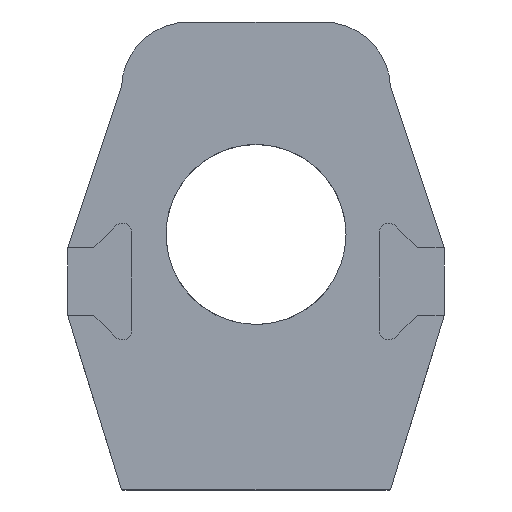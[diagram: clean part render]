
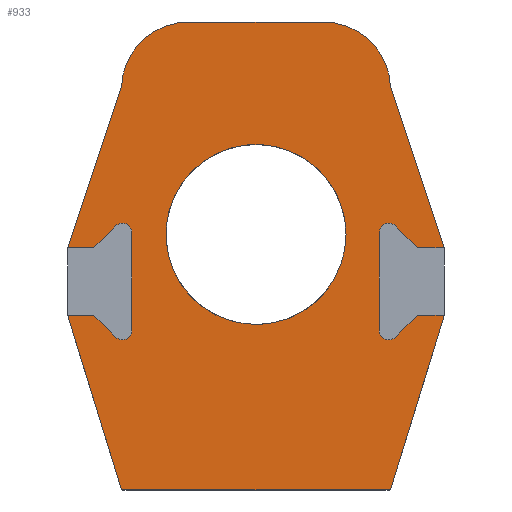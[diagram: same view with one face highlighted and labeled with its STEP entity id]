
A CAD part, front view. The second image highlights one B-rep face of the part: STEP entity #933.
In plain terms, the highlighted planar face has unit normal (0, -1, 0).
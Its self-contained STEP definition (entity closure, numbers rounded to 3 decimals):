
#19=ELLIPSE('',#1005,3.676,2.54);
#20=ELLIPSE('',#1012,3.676,2.54);
#58=FACE_BOUND('',#143,.T.);
#62=PLANE('',#1004);
#91=FACE_OUTER_BOUND('',#142,.T.);
#142=EDGE_LOOP('',(#667,#668,#669,#670,#671,#672,#673,#674,#675,#676,#677,
#678,#679,#680,#681,#682,#683,#684,#685,#686,#687,#688,#689,#690));
#143=EDGE_LOOP('',(#691,#692));
#202=LINE('',#1413,#299);
#203=LINE('',#1415,#300);
#204=LINE('',#1417,#301);
#205=LINE('',#1421,#302);
#206=LINE('',#1425,#303);
#207=LINE('',#1427,#304);
#208=LINE('',#1429,#305);
#209=LINE('',#1433,#306);
#210=LINE('',#1437,#307);
#211=LINE('',#1439,#308);
#212=LINE('',#1441,#309);
#213=LINE('',#1445,#310);
#214=LINE('',#1449,#311);
#215=LINE('',#1451,#312);
#216=LINE('',#1453,#313);
#217=LINE('',#1456,#314);
#299=VECTOR('',#1123,10.);
#300=VECTOR('',#1124,10.);
#301=VECTOR('',#1125,10.);
#302=VECTOR('',#1128,10.);
#303=VECTOR('',#1131,10.);
#304=VECTOR('',#1132,10.);
#305=VECTOR('',#1133,10.);
#306=VECTOR('',#1136,10.);
#307=VECTOR('',#1139,10.);
#308=VECTOR('',#1140,10.);
#309=VECTOR('',#1141,10.);
#310=VECTOR('',#1144,10.);
#311=VECTOR('',#1147,10.);
#312=VECTOR('',#1148,10.);
#313=VECTOR('',#1149,10.);
#314=VECTOR('',#1152,10.);
#393=CIRCLE('',#1006,0.889);
#394=CIRCLE('',#1007,0.889);
#395=CIRCLE('',#1008,6.35);
#396=CIRCLE('',#1009,6.35);
#397=CIRCLE('',#1010,0.889);
#398=CIRCLE('',#1011,0.889);
#399=CIRCLE('',#1013,8.5);
#400=CIRCLE('',#1014,8.5);
#426=VERTEX_POINT('',#1409);
#427=VERTEX_POINT('',#1410);
#428=VERTEX_POINT('',#1412);
#429=VERTEX_POINT('',#1414);
#430=VERTEX_POINT('',#1416);
#431=VERTEX_POINT('',#1418);
#432=VERTEX_POINT('',#1420);
#433=VERTEX_POINT('',#1422);
#434=VERTEX_POINT('',#1424);
#435=VERTEX_POINT('',#1426);
#436=VERTEX_POINT('',#1428);
#437=VERTEX_POINT('',#1430);
#438=VERTEX_POINT('',#1432);
#439=VERTEX_POINT('',#1434);
#440=VERTEX_POINT('',#1436);
#441=VERTEX_POINT('',#1438);
#442=VERTEX_POINT('',#1440);
#443=VERTEX_POINT('',#1442);
#444=VERTEX_POINT('',#1444);
#445=VERTEX_POINT('',#1446);
#446=VERTEX_POINT('',#1448);
#447=VERTEX_POINT('',#1450);
#448=VERTEX_POINT('',#1452);
#449=VERTEX_POINT('',#1454);
#450=VERTEX_POINT('',#1457);
#451=VERTEX_POINT('',#1458);
#520=EDGE_CURVE('',#426,#427,#19,.T.);
#521=EDGE_CURVE('',#426,#428,#202,.T.);
#522=EDGE_CURVE('',#429,#428,#203,.T.);
#523=EDGE_CURVE('',#430,#429,#204,.T.);
#524=EDGE_CURVE('',#431,#430,#393,.T.);
#525=EDGE_CURVE('',#432,#431,#205,.T.);
#526=EDGE_CURVE('',#433,#432,#394,.T.);
#527=EDGE_CURVE('',#434,#433,#206,.T.);
#528=EDGE_CURVE('',#435,#434,#207,.T.);
#529=EDGE_CURVE('',#435,#436,#208,.T.);
#530=EDGE_CURVE('',#436,#437,#395,.T.);
#531=EDGE_CURVE('',#437,#438,#209,.T.);
#532=EDGE_CURVE('',#438,#439,#396,.T.);
#533=EDGE_CURVE('',#439,#440,#210,.T.);
#534=EDGE_CURVE('',#441,#440,#211,.T.);
#535=EDGE_CURVE('',#442,#441,#212,.T.);
#536=EDGE_CURVE('',#443,#442,#397,.T.);
#537=EDGE_CURVE('',#444,#443,#213,.T.);
#538=EDGE_CURVE('',#445,#444,#398,.T.);
#539=EDGE_CURVE('',#446,#445,#214,.T.);
#540=EDGE_CURVE('',#447,#446,#215,.T.);
#541=EDGE_CURVE('',#447,#448,#216,.T.);
#542=EDGE_CURVE('',#449,#448,#20,.T.);
#543=EDGE_CURVE('',#449,#427,#217,.T.);
#544=EDGE_CURVE('',#450,#451,#399,.T.);
#545=EDGE_CURVE('',#451,#450,#400,.T.);
#667=ORIENTED_EDGE('',*,*,#520,.F.);
#668=ORIENTED_EDGE('',*,*,#521,.T.);
#669=ORIENTED_EDGE('',*,*,#522,.F.);
#670=ORIENTED_EDGE('',*,*,#523,.F.);
#671=ORIENTED_EDGE('',*,*,#524,.F.);
#672=ORIENTED_EDGE('',*,*,#525,.F.);
#673=ORIENTED_EDGE('',*,*,#526,.F.);
#674=ORIENTED_EDGE('',*,*,#527,.F.);
#675=ORIENTED_EDGE('',*,*,#528,.F.);
#676=ORIENTED_EDGE('',*,*,#529,.T.);
#677=ORIENTED_EDGE('',*,*,#530,.T.);
#678=ORIENTED_EDGE('',*,*,#531,.T.);
#679=ORIENTED_EDGE('',*,*,#532,.T.);
#680=ORIENTED_EDGE('',*,*,#533,.T.);
#681=ORIENTED_EDGE('',*,*,#534,.F.);
#682=ORIENTED_EDGE('',*,*,#535,.F.);
#683=ORIENTED_EDGE('',*,*,#536,.F.);
#684=ORIENTED_EDGE('',*,*,#537,.F.);
#685=ORIENTED_EDGE('',*,*,#538,.F.);
#686=ORIENTED_EDGE('',*,*,#539,.F.);
#687=ORIENTED_EDGE('',*,*,#540,.F.);
#688=ORIENTED_EDGE('',*,*,#541,.T.);
#689=ORIENTED_EDGE('',*,*,#542,.F.);
#690=ORIENTED_EDGE('',*,*,#543,.T.);
#691=ORIENTED_EDGE('',*,*,#544,.T.);
#692=ORIENTED_EDGE('',*,*,#545,.T.);
#933=ADVANCED_FACE('',(#91,#58),#62,.F.);
#1004=AXIS2_PLACEMENT_3D('',#1408,#1119,#1120);
#1005=AXIS2_PLACEMENT_3D('',#1411,#1121,#1122);
#1006=AXIS2_PLACEMENT_3D('',#1419,#1126,#1127);
#1007=AXIS2_PLACEMENT_3D('',#1423,#1129,#1130);
#1008=AXIS2_PLACEMENT_3D('',#1431,#1134,#1135);
#1009=AXIS2_PLACEMENT_3D('',#1435,#1137,#1138);
#1010=AXIS2_PLACEMENT_3D('',#1443,#1142,#1143);
#1011=AXIS2_PLACEMENT_3D('',#1447,#1145,#1146);
#1012=AXIS2_PLACEMENT_3D('',#1455,#1150,#1151);
#1013=AXIS2_PLACEMENT_3D('',#1459,#1153,#1154);
#1014=AXIS2_PLACEMENT_3D('',#1460,#1155,#1156);
#1119=DIRECTION('center_axis',(0.,1.,0.));
#1120=DIRECTION('ref_axis',(-1.,0.,0.));
#1121=DIRECTION('center_axis',(0.,1.,0.));
#1122=DIRECTION('ref_axis',(-0.294,0.,-0.956));
#1123=DIRECTION('',(0.294,0.,0.956));
#1124=DIRECTION('',(1.,0.,0.));
#1125=DIRECTION('',(0.707,0.,0.707));
#1126=DIRECTION('center_axis',(0.,-1.,0.));
#1127=DIRECTION('ref_axis',(0.707,0.,-0.707));
#1128=DIRECTION('',(0.,0.,-1.));
#1129=DIRECTION('center_axis',(0.,-1.,0.));
#1130=DIRECTION('ref_axis',(-1.,0.,0.));
#1131=DIRECTION('',(-0.707,0.,0.707));
#1132=DIRECTION('',(-1.,0.,0.001));
#1133=DIRECTION('',(-0.316,0.,0.949));
#1134=DIRECTION('center_axis',(0.,-1.,0.));
#1135=DIRECTION('ref_axis',(0.999,0.,0.04));
#1136=DIRECTION('',(-1.,0.,0.));
#1137=DIRECTION('center_axis',(0.,-1.,0.));
#1138=DIRECTION('ref_axis',(-0.999,0.,0.04));
#1139=DIRECTION('',(-0.316,0.,-0.949));
#1140=DIRECTION('',(-1.,0.,-0.001));
#1141=DIRECTION('',(-0.707,0.,-0.707));
#1142=DIRECTION('center_axis',(0.,-1.,0.));
#1143=DIRECTION('ref_axis',(-0.707,0.,0.707));
#1144=DIRECTION('',(0.,0.,1.));
#1145=DIRECTION('center_axis',(0.,-1.,0.));
#1146=DIRECTION('ref_axis',(1.,0.,0.));
#1147=DIRECTION('',(0.707,0.,-0.707));
#1148=DIRECTION('',(1.,0.,0.));
#1149=DIRECTION('',(0.294,0.,-0.956));
#1150=DIRECTION('center_axis',(0.,1.,0.));
#1151=DIRECTION('ref_axis',(0.294,0.,-0.956));
#1152=DIRECTION('',(1.,0.,0.));
#1153=DIRECTION('center_axis',(0.,1.,0.));
#1154=DIRECTION('ref_axis',(-1.,0.,0.));
#1155=DIRECTION('center_axis',(0.,1.,0.));
#1156=DIRECTION('ref_axis',(-1.,0.,0.));
#1408=CARTESIAN_POINT('Origin',(0.,171.04,6.35));
#1409=CARTESIAN_POINT('',(12.794,171.04,-12.394));
#1410=CARTESIAN_POINT('',(12.69,171.04,-12.699));
#1411=CARTESIAN_POINT('Origin',(10.366,171.04,-11.647));
#1412=CARTESIAN_POINT('',(17.78,171.04,3.81));
#1413=CARTESIAN_POINT('',(17.368,171.04,2.471));
#1414=CARTESIAN_POINT('',(15.24,171.04,3.81));
#1415=CARTESIAN_POINT('',(8.89,171.04,3.81));
#1416=CARTESIAN_POINT('',(13.166,171.04,1.736));
#1417=CARTESIAN_POINT('',(12.065,171.04,0.635));
#1418=CARTESIAN_POINT('',(11.648,171.04,2.364));
#1419=CARTESIAN_POINT('Origin',(12.537,171.04,2.364));
#1420=CARTESIAN_POINT('',(11.648,171.04,11.609));
#1421=CARTESIAN_POINT('',(11.648,171.04,4.357));
#1422=CARTESIAN_POINT('',(13.166,171.04,12.238));
#1423=CARTESIAN_POINT('Origin',(12.537,171.04,11.609));
#1424=CARTESIAN_POINT('',(15.24,171.04,10.163));
#1425=CARTESIAN_POINT('',(11.346,171.04,14.057));
#1426=CARTESIAN_POINT('',(17.78,171.04,10.16));
#1427=CARTESIAN_POINT('',(7.622,171.04,10.172));
#1428=CARTESIAN_POINT('',(12.7,171.04,25.4));
#1429=CARTESIAN_POINT('',(14.923,171.04,18.733));
#1430=CARTESIAN_POINT('',(6.355,171.04,31.496));
#1431=CARTESIAN_POINT('Origin',(6.355,171.04,25.146));
#1432=CARTESIAN_POINT('',(-6.355,171.04,31.496));
#1433=CARTESIAN_POINT('',(-6.35,171.04,31.496));
#1434=CARTESIAN_POINT('',(-12.7,171.04,25.4));
#1435=CARTESIAN_POINT('Origin',(-6.355,171.04,25.146));
#1436=CARTESIAN_POINT('',(-17.78,171.04,10.16));
#1437=CARTESIAN_POINT('',(-17.463,171.04,11.113));
#1438=CARTESIAN_POINT('',(-15.317,171.04,10.163));
#1439=CARTESIAN_POINT('',(-8.892,171.04,10.171));
#1440=CARTESIAN_POINT('',(-13.243,171.04,12.238));
#1441=CARTESIAN_POINT('',(-12.441,171.04,13.039));
#1442=CARTESIAN_POINT('',(-11.725,171.04,11.609));
#1443=CARTESIAN_POINT('Origin',(-12.614,171.04,11.609));
#1444=CARTESIAN_POINT('',(-11.725,171.04,2.364));
#1445=CARTESIAN_POINT('',(-11.725,171.04,8.979));
#1446=CARTESIAN_POINT('',(-13.243,171.04,1.736));
#1447=CARTESIAN_POINT('Origin',(-12.614,171.04,2.364));
#1448=CARTESIAN_POINT('',(-15.317,171.04,3.81));
#1449=CARTESIAN_POINT('',(-11.086,171.04,-0.422));
#1450=CARTESIAN_POINT('',(-17.78,171.04,3.81));
#1451=CARTESIAN_POINT('',(-7.659,171.04,3.81));
#1452=CARTESIAN_POINT('',(-12.794,171.04,-12.394));
#1453=CARTESIAN_POINT('',(-14.828,171.04,-5.784));
#1454=CARTESIAN_POINT('',(-12.69,171.04,-12.699));
#1455=CARTESIAN_POINT('Origin',(-10.366,171.04,-11.647));
#1456=CARTESIAN_POINT('',(6.35,171.04,-12.699));
#1457=CARTESIAN_POINT('',(8.064,171.04,14.118));
#1458=CARTESIAN_POINT('',(8.5,171.04,11.43));
#1459=CARTESIAN_POINT('Origin',(0.,171.04,11.43));
#1460=CARTESIAN_POINT('Origin',(0.,171.04,11.43));
